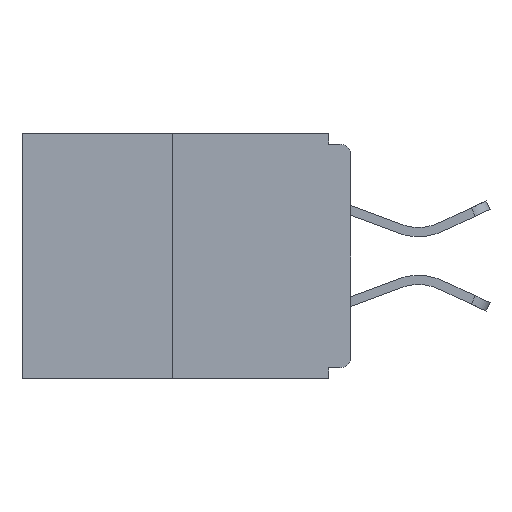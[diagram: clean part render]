
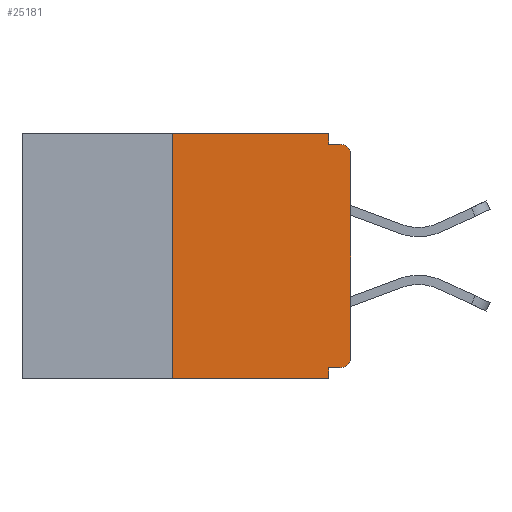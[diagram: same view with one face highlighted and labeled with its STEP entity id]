
A CAD part, left-side view. The second image highlights one B-rep face of the part: STEP entity #25181.
In plain terms, the highlighted planar face has unit normal (-1, 0, 0).
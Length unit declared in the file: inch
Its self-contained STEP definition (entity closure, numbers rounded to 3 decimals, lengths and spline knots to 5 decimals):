
#206 = ORIENTED_EDGE ( 'NONE', *, *, #22974, .T. ) ;
#1058 = LINE ( 'NONE', #4469, #23013 ) ;
#1406 = ORIENTED_EDGE ( 'NONE', *, *, #19110, .F. ) ;
#1598 = EDGE_CURVE ( 'NONE', #15534, #10549, #1058, .T. ) ;
#2542 = VERTEX_POINT ( 'NONE', #26315 ) ;
#2644 = EDGE_CURVE ( 'NONE', #2542, #21109, #18914, .T. ) ;
#3306 = CARTESIAN_POINT ( 'NONE',  ( 0., 0., -0.313 ) ) ;
#3953 = CARTESIAN_POINT ( 'NONE',  ( 0., 0.46, 0. ) ) ;
#4252 = VERTEX_POINT ( 'NONE', #26038 ) ;
#4469 = CARTESIAN_POINT ( 'NONE',  ( 0., 0., 0. ) ) ;
#4496 = LINE ( 'NONE', #3953, #24770 ) ;
#4696 = EDGE_CURVE ( 'NONE', #15283, #21109, #12503, .T. ) ;
#6208 = FACE_OUTER_BOUND ( 'NONE', #22400, .T. ) ;
#6260 = CARTESIAN_POINT ( 'NONE',  ( 0., 0.25, 0. ) ) ;
#6698 = ORIENTED_EDGE ( 'NONE', *, *, #21475, .T. ) ;
#6709 = AXIS2_PLACEMENT_3D ( 'NONE', #11853, #26650, #18515 ) ;
#6716 = DIRECTION ( 'NONE',  ( 0., 0., 1. ) ) ;
#6786 = CIRCLE ( 'NONE', #9862, 0.015 ) ;
#6865 = DIRECTION ( 'NONE',  ( 0., 0., -1. ) ) ;
#7521 = CARTESIAN_POINT ( 'NONE',  ( 0., 0., -0.328 ) ) ;
#8129 = DIRECTION ( 'NONE',  ( 0., 0., -1. ) ) ;
#8393 = CARTESIAN_POINT ( 'NONE',  ( 0., 0.031, 0. ) ) ;
#9862 = AXIS2_PLACEMENT_3D ( 'NONE', #13357, #19556, #25948 ) ;
#10262 = DIRECTION ( 'NONE',  ( 0., 0., -1. ) ) ;
#10445 = DIRECTION ( 'NONE',  ( 0., 0., 1. ) ) ;
#10549 = VERTEX_POINT ( 'NONE', #18356 ) ;
#10778 = ORIENTED_EDGE ( 'NONE', *, *, #2644, .T. ) ;
#11297 = VERTEX_POINT ( 'NONE', #25674 ) ;
#11336 = CARTESIAN_POINT ( 'NONE',  ( 0., 0.031, -0.015 ) ) ;
#11595 = CARTESIAN_POINT ( 'NONE',  ( 0., 0.25, 0. ) ) ;
#11853 = CARTESIAN_POINT ( 'NONE',  ( 0., 0.46, 0. ) ) ;
#11879 = ORIENTED_EDGE ( 'NONE', *, *, #22619, .F. ) ;
#12434 = LINE ( 'NONE', #6260, #13412 ) ;
#12503 = LINE ( 'NONE', #13206, #27408 ) ;
#13206 = CARTESIAN_POINT ( 'NONE',  ( 0., 0.031, -0.343 ) ) ;
#13211 = LINE ( 'NONE', #8393, #22180 ) ;
#13357 = CARTESIAN_POINT ( 'NONE',  ( 0., 0.015, -0.313 ) ) ;
#13412 = VECTOR ( 'NONE', #10445, 39.37008 ) ;
#13469 = EDGE_CURVE ( 'NONE', #4252, #16427, #13211, .T. ) ;
#13813 = DIRECTION ( 'NONE',  ( 0., -1., 0. ) ) ;
#14537 = EDGE_CURVE ( 'NONE', #22508, #4252, #4496, .T. ) ;
#14819 = DIRECTION ( 'NONE',  ( -1., 0., 0. ) ) ;
#15174 = ORIENTED_EDGE ( 'NONE', *, *, #13469, .F. ) ;
#15283 = VERTEX_POINT ( 'NONE', #19405 ) ;
#15534 = VERTEX_POINT ( 'NONE', #3306 ) ;
#16134 = CARTESIAN_POINT ( 'NONE',  ( 0., 0., -0.015 ) ) ;
#16270 = VECTOR ( 'NONE', #13813, 39.37008 ) ;
#16427 = VERTEX_POINT ( 'NONE', #11336 ) ;
#16522 = DIRECTION ( 'NONE',  ( 0., -1., 0. ) ) ;
#16796 = LINE ( 'NONE', #16134, #26046 ) ;
#17433 = ORIENTED_EDGE ( 'NONE', *, *, #4696, .F. ) ;
#18356 = CARTESIAN_POINT ( 'NONE',  ( 0., 0., -0.03 ) ) ;
#18515 = DIRECTION ( 'NONE',  ( 0., 0., -1. ) ) ;
#18682 = CARTESIAN_POINT ( 'NONE',  ( 0., 0.015, -0.328 ) ) ;
#18914 = LINE ( 'NONE', #26759, #16270 ) ;
#19110 = EDGE_CURVE ( 'NONE', #23512, #15283, #21337, .T. ) ;
#19405 = CARTESIAN_POINT ( 'NONE',  ( 0., 0.031, -0.328 ) ) ;
#19556 = DIRECTION ( 'NONE',  ( -1., 0., 0. ) ) ;
#20194 = DIRECTION ( 'NONE',  ( 0., -1., 0. ) ) ;
#20701 = AXIS2_PLACEMENT_3D ( 'NONE', #27314, #14819, #8129 ) ;
#21109 = VERTEX_POINT ( 'NONE', #26591 ) ;
#21337 = LINE ( 'NONE', #7521, #25258 ) ;
#21411 = ORIENTED_EDGE ( 'NONE', *, *, #27020, .F. ) ;
#21464 = ORIENTED_EDGE ( 'NONE', *, *, #1598, .T. ) ;
#21475 = EDGE_CURVE ( 'NONE', #10549, #11297, #21518, .T. ) ;
#21518 = CIRCLE ( 'NONE', #20701, 0.015 ) ;
#22180 = VECTOR ( 'NONE', #10262, 39.37008 ) ;
#22214 = DIRECTION ( 'NONE',  ( 0., 1., 0. ) ) ;
#22400 = EDGE_LOOP ( 'NONE', ( #22770, #21411, #10778, #17433, #1406, #206, #21464, #6698, #11879, #15174 ) ) ;
#22426 = PLANE ( 'NONE',  #6709 ) ;
#22508 = VERTEX_POINT ( 'NONE', #11595 ) ;
#22619 = EDGE_CURVE ( 'NONE', #16427, #11297, #16796, .T. ) ;
#22770 = ORIENTED_EDGE ( 'NONE', *, *, #14537, .F. ) ;
#22974 = EDGE_CURVE ( 'NONE', #23512, #15534, #6786, .T. ) ;
#23013 = VECTOR ( 'NONE', #6716, 39.37008 ) ;
#23512 = VERTEX_POINT ( 'NONE', #18682 ) ;
#24770 = VECTOR ( 'NONE', #16522, 39.37008 ) ;
#25181 = ADVANCED_FACE ( 'NONE', ( #6208 ), #22426, .F. ) ;
#25258 = VECTOR ( 'NONE', #22214, 39.37008 ) ;
#25674 = CARTESIAN_POINT ( 'NONE',  ( 0., 0.015, -0.015 ) ) ;
#25948 = DIRECTION ( 'NONE',  ( 0., 0., -1. ) ) ;
#26038 = CARTESIAN_POINT ( 'NONE',  ( 0., 0.031, 0. ) ) ;
#26046 = VECTOR ( 'NONE', #20194, 39.37008 ) ;
#26315 = CARTESIAN_POINT ( 'NONE',  ( 0., 0.25, -0.343 ) ) ;
#26591 = CARTESIAN_POINT ( 'NONE',  ( 0., 0.031, -0.343 ) ) ;
#26650 = DIRECTION ( 'NONE',  ( 1., 0., 0. ) ) ;
#26759 = CARTESIAN_POINT ( 'NONE',  ( 0., 0.46, -0.343 ) ) ;
#27020 = EDGE_CURVE ( 'NONE', #2542, #22508, #12434, .T. ) ;
#27314 = CARTESIAN_POINT ( 'NONE',  ( 0., 0.015, -0.03 ) ) ;
#27408 = VECTOR ( 'NONE', #6865, 39.37008 ) ;
